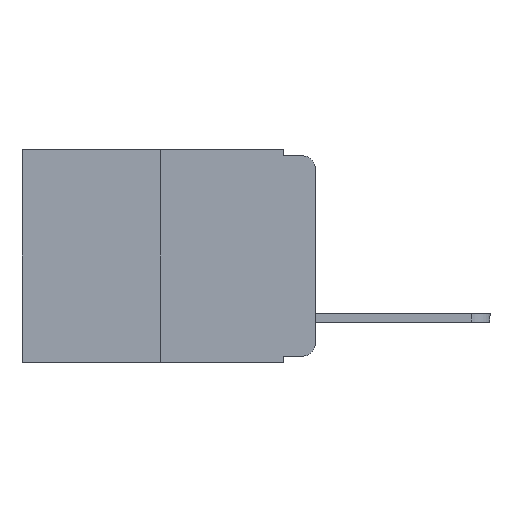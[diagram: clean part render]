
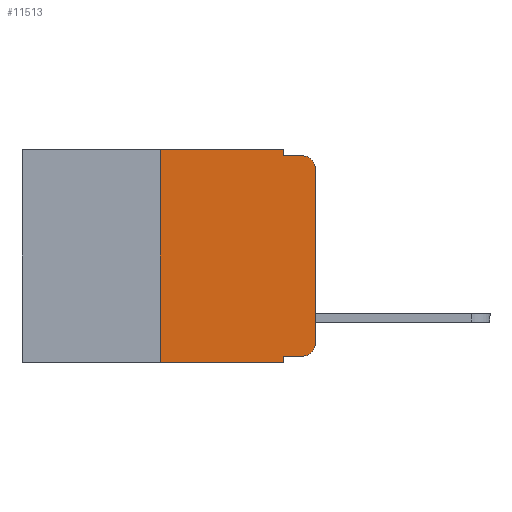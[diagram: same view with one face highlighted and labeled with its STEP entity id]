
A CAD part, left-side view. The second image highlights one B-rep face of the part: STEP entity #11513.
In plain terms, the highlighted planar face has unit normal (-1, 0, 0).
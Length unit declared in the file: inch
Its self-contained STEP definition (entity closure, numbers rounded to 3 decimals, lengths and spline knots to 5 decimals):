
#68 = DIRECTION ( 'NONE',  ( 0., -1., 0. ) ) ;
#211 = CARTESIAN_POINT ( 'NONE',  ( 0., 0.25, -0.343 ) ) ;
#292 = VECTOR ( 'NONE', #2436, 39.37008 ) ;
#666 = CARTESIAN_POINT ( 'NONE',  ( 0., 0.02, -0.01 ) ) ;
#729 = LINE ( 'NONE', #15763, #292 ) ;
#822 = VERTEX_POINT ( 'NONE', #17065 ) ;
#1179 = CARTESIAN_POINT ( 'NONE',  ( 0., 0.051, 0. ) ) ;
#1351 = EDGE_CURVE ( 'NONE', #5278, #5089, #16630, .T. ) ;
#1402 = VERTEX_POINT ( 'NONE', #9591 ) ;
#1460 = DIRECTION ( 'NONE',  ( 0., 0., 1. ) ) ;
#1692 = DIRECTION ( 'NONE',  ( -1., 0., 0. ) ) ;
#1844 = EDGE_CURVE ( 'NONE', #12540, #9975, #15812, .T. ) ;
#1935 = CARTESIAN_POINT ( 'NONE',  ( 0., 0., -0.03 ) ) ;
#2436 = DIRECTION ( 'NONE',  ( 0., 0., -1. ) ) ;
#2471 = VERTEX_POINT ( 'NONE', #1179 ) ;
#2827 = DIRECTION ( 'NONE',  ( 0., 0., 1. ) ) ;
#2854 = VERTEX_POINT ( 'NONE', #13672 ) ;
#3052 = DIRECTION ( 'NONE',  ( 1., 0., 0. ) ) ;
#3082 = DIRECTION ( 'NONE',  ( 0., 0., -1. ) ) ;
#3096 = ORIENTED_EDGE ( 'NONE', *, *, #16696, .T. ) ;
#3353 = LINE ( 'NONE', #11558, #13657 ) ;
#3754 = CARTESIAN_POINT ( 'NONE',  ( 0., 0.051, -0.343 ) ) ;
#3925 = CARTESIAN_POINT ( 'NONE',  ( 0., 0.051, -0.333 ) ) ;
#4520 = CARTESIAN_POINT ( 'NONE',  ( 0., 0.02, -0.313 ) ) ;
#4973 = DIRECTION ( 'NONE',  ( 0., -1., 0. ) ) ;
#5089 = VERTEX_POINT ( 'NONE', #3754 ) ;
#5278 = VERTEX_POINT ( 'NONE', #211 ) ;
#5423 = AXIS2_PLACEMENT_3D ( 'NONE', #9835, #1692, #11181 ) ;
#5554 = EDGE_CURVE ( 'NONE', #5278, #2854, #9592, .T. ) ;
#5711 = CARTESIAN_POINT ( 'NONE',  ( 0., 0.473, 0. ) ) ;
#5872 = DIRECTION ( 'NONE',  ( 0., 0., -1. ) ) ;
#6328 = AXIS2_PLACEMENT_3D ( 'NONE', #5711, #3052, #12468 ) ;
#6491 = DIRECTION ( 'NONE',  ( 0., -1., 0. ) ) ;
#6947 = CARTESIAN_POINT ( 'NONE',  ( 0., 0.051, -0.01 ) ) ;
#7084 = PLANE ( 'NONE',  #6328 ) ;
#7113 = CARTESIAN_POINT ( 'NONE',  ( 0., 0.051, 0. ) ) ;
#7140 = CARTESIAN_POINT ( 'NONE',  ( 0., 0.051, -0.333 ) ) ;
#7333 = ORIENTED_EDGE ( 'NONE', *, *, #7807, .F. ) ;
#7807 = EDGE_CURVE ( 'NONE', #2471, #1402, #15303, .T. ) ;
#7922 = CARTESIAN_POINT ( 'NONE',  ( 0., 0.25, 0. ) ) ;
#7992 = VERTEX_POINT ( 'NONE', #666 ) ;
#8603 = VECTOR ( 'NONE', #1460, 39.37008 ) ;
#8788 = VECTOR ( 'NONE', #6491, 39.37008 ) ;
#9008 = ORIENTED_EDGE ( 'NONE', *, *, #1351, .T. ) ;
#9067 = CIRCLE ( 'NONE', #10588, 0.02 ) ;
#9457 = FACE_OUTER_BOUND ( 'NONE', #16192, .T. ) ;
#9591 = CARTESIAN_POINT ( 'NONE',  ( 0., 0.051, -0.01 ) ) ;
#9592 = LINE ( 'NONE', #7922, #16175 ) ;
#9626 = CARTESIAN_POINT ( 'NONE',  ( 0., 0., 0. ) ) ;
#9835 = CARTESIAN_POINT ( 'NONE',  ( 0., 0.02, -0.03 ) ) ;
#9975 = VERTEX_POINT ( 'NONE', #11820 ) ;
#10401 = CARTESIAN_POINT ( 'NONE',  ( 0., 0.473, -0.343 ) ) ;
#10588 = AXIS2_PLACEMENT_3D ( 'NONE', #4520, #13896, #5872 ) ;
#10903 = ORIENTED_EDGE ( 'NONE', *, *, #12367, .F. ) ;
#11181 = DIRECTION ( 'NONE',  ( 0., 0., -1. ) ) ;
#11513 = ADVANCED_FACE ( 'NONE', ( #9457 ), #7084, .F. ) ;
#11524 = EDGE_CURVE ( 'NONE', #15737, #7992, #15653, .T. ) ;
#11558 = CARTESIAN_POINT ( 'NONE',  ( 0., 0.473, 0. ) ) ;
#11574 = LINE ( 'NONE', #6947, #13003 ) ;
#11820 = CARTESIAN_POINT ( 'NONE',  ( 0., 0.02, -0.333 ) ) ;
#12094 = EDGE_CURVE ( 'NONE', #1402, #7992, #11574, .T. ) ;
#12180 = LINE ( 'NONE', #9626, #8603 ) ;
#12357 = ORIENTED_EDGE ( 'NONE', *, *, #12649, .T. ) ;
#12367 = EDGE_CURVE ( 'NONE', #2854, #2471, #3353, .T. ) ;
#12468 = DIRECTION ( 'NONE',  ( 0., 0., -1. ) ) ;
#12540 = VERTEX_POINT ( 'NONE', #3925 ) ;
#12649 = EDGE_CURVE ( 'NONE', #822, #15737, #12180, .T. ) ;
#12762 = ORIENTED_EDGE ( 'NONE', *, *, #11524, .T. ) ;
#12780 = VECTOR ( 'NONE', #4973, 39.37008 ) ;
#12984 = ORIENTED_EDGE ( 'NONE', *, *, #15911, .F. ) ;
#13003 = VECTOR ( 'NONE', #68, 39.37008 ) ;
#13657 = VECTOR ( 'NONE', #14232, 39.37008 ) ;
#13672 = CARTESIAN_POINT ( 'NONE',  ( 0., 0.25, 0. ) ) ;
#13896 = DIRECTION ( 'NONE',  ( -1., 0., 0. ) ) ;
#14232 = DIRECTION ( 'NONE',  ( 0., -1., 0. ) ) ;
#14834 = ORIENTED_EDGE ( 'NONE', *, *, #5554, .F. ) ;
#14910 = VECTOR ( 'NONE', #3082, 39.37008 ) ;
#15303 = LINE ( 'NONE', #7113, #14910 ) ;
#15653 = CIRCLE ( 'NONE', #5423, 0.02 ) ;
#15737 = VERTEX_POINT ( 'NONE', #1935 ) ;
#15763 = CARTESIAN_POINT ( 'NONE',  ( 0., 0.051, 0. ) ) ;
#15812 = LINE ( 'NONE', #7140, #8788 ) ;
#15911 = EDGE_CURVE ( 'NONE', #12540, #5089, #729, .T. ) ;
#16175 = VECTOR ( 'NONE', #2827, 39.37008 ) ;
#16192 = EDGE_LOOP ( 'NONE', ( #12357, #12762, #17032, #7333, #10903, #14834, #9008, #12984, #16412, #3096 ) ) ;
#16412 = ORIENTED_EDGE ( 'NONE', *, *, #1844, .T. ) ;
#16630 = LINE ( 'NONE', #10401, #12780 ) ;
#16696 = EDGE_CURVE ( 'NONE', #9975, #822, #9067, .T. ) ;
#17032 = ORIENTED_EDGE ( 'NONE', *, *, #12094, .F. ) ;
#17065 = CARTESIAN_POINT ( 'NONE',  ( 0., 0., -0.313 ) ) ;
